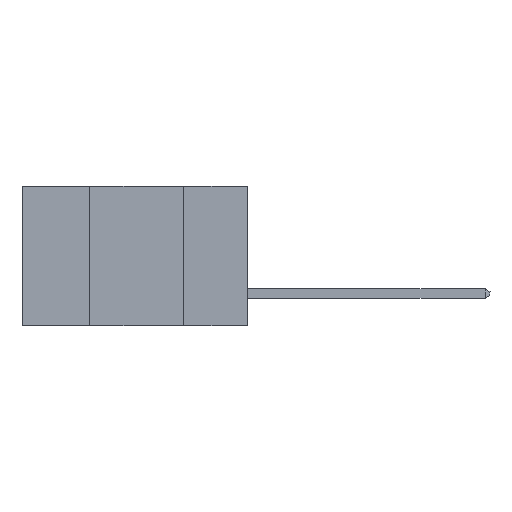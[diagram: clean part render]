
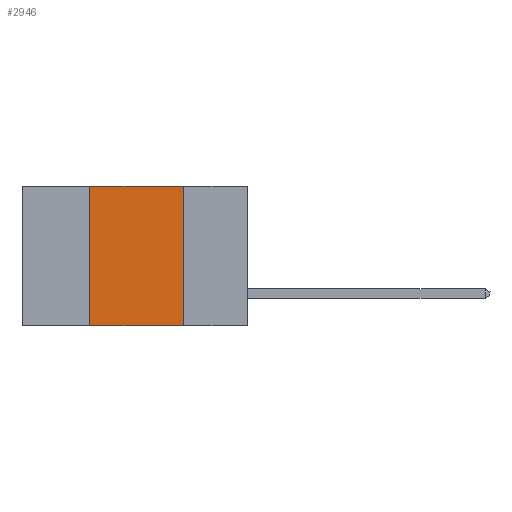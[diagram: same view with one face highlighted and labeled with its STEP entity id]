
A CAD part, left-side view. The second image highlights one B-rep face of the part: STEP entity #2946.
In plain terms, the highlighted planar face has unit normal (-1, 0, 0).
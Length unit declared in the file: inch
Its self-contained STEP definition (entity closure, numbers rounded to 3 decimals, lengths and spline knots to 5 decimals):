
#587 = CARTESIAN_POINT ( 'NONE',  ( 0., 0.6, -0.37 ) ) ;
#1130 = CARTESIAN_POINT ( 'NONE',  ( 0., 0.42, -0.37 ) ) ;
#1295 = ORIENTED_EDGE ( 'NONE', *, *, #8039, .F. ) ;
#1491 = DIRECTION ( 'NONE',  ( 1., 0., 0. ) ) ;
#1841 = LINE ( 'NONE', #7542, #10396 ) ;
#2093 = ORIENTED_EDGE ( 'NONE', *, *, #10455, .F. ) ;
#2286 = EDGE_LOOP ( 'NONE', ( #2093, #6662, #1295, #10377 ) ) ;
#2378 = VERTEX_POINT ( 'NONE', #1130 ) ;
#2946 = ADVANCED_FACE ( 'NONE', ( #7976 ), #3065, .F. ) ;
#3065 = PLANE ( 'NONE',  #5577 ) ;
#3174 = DIRECTION ( 'NONE',  ( 0., -1., 0. ) ) ;
#3280 = DIRECTION ( 'NONE',  ( 0., 0., 1. ) ) ;
#3607 = VERTEX_POINT ( 'NONE', #3726 ) ;
#3726 = CARTESIAN_POINT ( 'NONE',  ( 0., 0.17, 0. ) ) ;
#3769 = CARTESIAN_POINT ( 'NONE',  ( 0., 0.6, 0. ) ) ;
#3852 = VECTOR ( 'NONE', #10483, 39.37008 ) ;
#4826 = VERTEX_POINT ( 'NONE', #7416 ) ;
#5050 = DIRECTION ( 'NONE',  ( 0., 0., -1. ) ) ;
#5431 = VECTOR ( 'NONE', #3174, 39.37008 ) ;
#5577 = AXIS2_PLACEMENT_3D ( 'NONE', #3769, #1491, #6364 ) ;
#5653 = LINE ( 'NONE', #10638, #3852 ) ;
#6364 = DIRECTION ( 'NONE',  ( 0., 0., -1. ) ) ;
#6662 = ORIENTED_EDGE ( 'NONE', *, *, #7751, .F. ) ;
#7416 = CARTESIAN_POINT ( 'NONE',  ( 0., 0.17, -0.37 ) ) ;
#7524 = CARTESIAN_POINT ( 'NONE',  ( 0., 0.17, -0.37 ) ) ;
#7542 = CARTESIAN_POINT ( 'NONE',  ( 0., 0.42, -0.37 ) ) ;
#7693 = VECTOR ( 'NONE', #5050, 39.37008 ) ;
#7751 = EDGE_CURVE ( 'NONE', #10098, #3607, #5653, .T. ) ;
#7915 = EDGE_CURVE ( 'NONE', #2378, #4826, #10549, .T. ) ;
#7976 = FACE_OUTER_BOUND ( 'NONE', #2286, .T. ) ;
#8039 = EDGE_CURVE ( 'NONE', #2378, #10098, #1841, .T. ) ;
#9248 = LINE ( 'NONE', #7524, #7693 ) ;
#9370 = CARTESIAN_POINT ( 'NONE',  ( 0., 0.42, 0. ) ) ;
#10098 = VERTEX_POINT ( 'NONE', #9370 ) ;
#10377 = ORIENTED_EDGE ( 'NONE', *, *, #7915, .T. ) ;
#10396 = VECTOR ( 'NONE', #3280, 39.37008 ) ;
#10455 = EDGE_CURVE ( 'NONE', #3607, #4826, #9248, .T. ) ;
#10483 = DIRECTION ( 'NONE',  ( 0., -1., 0. ) ) ;
#10549 = LINE ( 'NONE', #587, #5431 ) ;
#10638 = CARTESIAN_POINT ( 'NONE',  ( 0., 0.6, 0. ) ) ;
